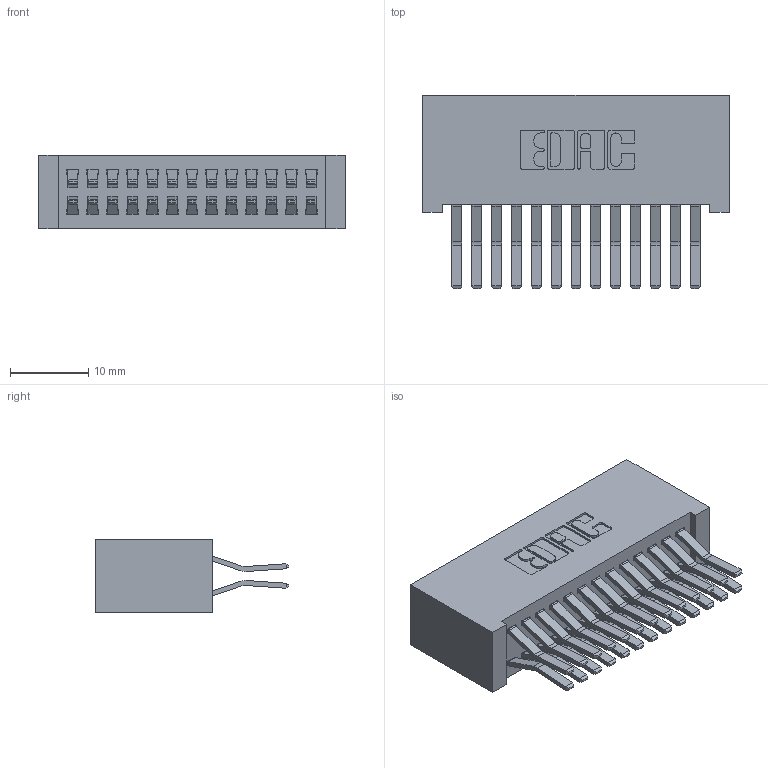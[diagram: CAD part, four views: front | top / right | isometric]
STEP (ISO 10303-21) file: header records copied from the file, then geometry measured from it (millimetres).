
FILE_DESCRIPTION (( 'STEP AP203' ), '1' );
FILE_NAME ('392-026-560-201.STEP', '2018-08-15T20:15:45', ( '' ), ( '' ), 'SwSTEP 2.0', 'SolidWorks 2016', '' );
FILE_SCHEMA (( 'CONFIG_CONTROL_DESIGN' ));
Length unit declared in the file: inch
Products named in the file (3): 342 Part_Lugless; 345-292-001_560 Tail; 392-026-560-201
Assembly tree (27 placements, depth 2):
  392-026-560-201
    342 Part_Lugless
    345-292-001_560 Tail  x26
Bounding box: 39.27 x 24.78 x 9.4 mm (x, y, z)
Volume: 4001.2 mm3; surface area: 6653.9 mm2
Topology: 27 solids, 27 shells, 1506 faces, 4461 edges, 2938 vertices
Faces by surface type: plane 998, cylinder 508
Entity records: 11793 total; most frequent: CARTESIAN_POINT 1986, ORIENTED_EDGE 1922, DIRECTION 1745, EDGE_CURVE 961, VECTOR 837, LINE 837, VERTEX_POINT 638, AXIS2_PLACEMENT_3D 454
